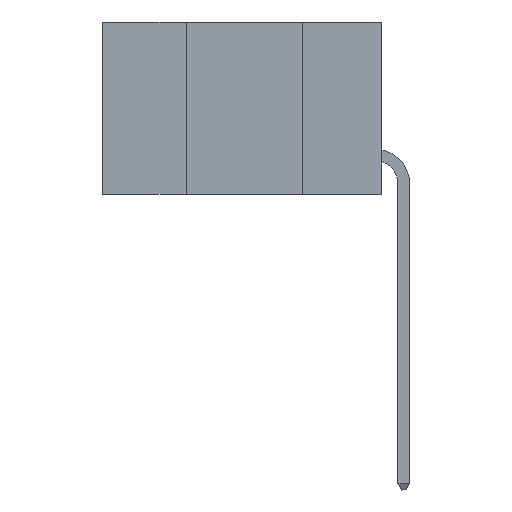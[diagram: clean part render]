
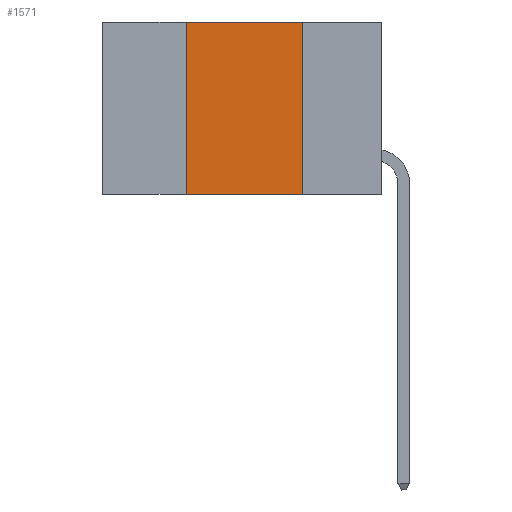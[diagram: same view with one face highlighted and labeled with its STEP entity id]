
A CAD part, left-side view. The second image highlights one B-rep face of the part: STEP entity #1571.
In plain terms, the highlighted planar face has unit normal (-1, 0, 0).
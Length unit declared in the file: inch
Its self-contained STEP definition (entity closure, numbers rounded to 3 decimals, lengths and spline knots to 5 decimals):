
#367 = CARTESIAN_POINT ( 'NONE',  ( 0., 0.6, -0.37 ) ) ;
#556 = VECTOR ( 'NONE', #1005, 39.37008 ) ;
#877 = DIRECTION ( 'NONE',  ( 0., -1., 0. ) ) ;
#901 = PLANE ( 'NONE',  #9043 ) ;
#1005 = DIRECTION ( 'NONE',  ( 0., 0., -1. ) ) ;
#1055 = EDGE_CURVE ( 'NONE', #2250, #11367, #5866, .T. ) ;
#1189 = ORIENTED_EDGE ( 'NONE', *, *, #10576, .F. ) ;
#1543 = ORIENTED_EDGE ( 'NONE', *, *, #1055, .F. ) ;
#1571 = ADVANCED_FACE ( 'NONE', ( #2139 ), #901, .F. ) ;
#1970 = LINE ( 'NONE', #11262, #9979 ) ;
#2139 = FACE_OUTER_BOUND ( 'NONE', #10655, .T. ) ;
#2250 = VERTEX_POINT ( 'NONE', #4619 ) ;
#2549 = ORIENTED_EDGE ( 'NONE', *, *, #5636, .F. ) ;
#2704 = DIRECTION ( 'NONE',  ( 0., 0., -1. ) ) ;
#2835 = VERTEX_POINT ( 'NONE', #10573 ) ;
#3587 = DIRECTION ( 'NONE',  ( 1., 0., 0. ) ) ;
#3677 = CARTESIAN_POINT ( 'NONE',  ( 0., 0.17, 0. ) ) ;
#3863 = LINE ( 'NONE', #10539, #556 ) ;
#4139 = EDGE_CURVE ( 'NONE', #2835, #9492, #4580, .T. ) ;
#4580 = LINE ( 'NONE', #367, #11360 ) ;
#4619 = CARTESIAN_POINT ( 'NONE',  ( 0., 0.42, 0. ) ) ;
#4703 = DIRECTION ( 'NONE',  ( 0., -1., 0. ) ) ;
#5636 = EDGE_CURVE ( 'NONE', #11367, #9492, #3863, .T. ) ;
#5839 = DIRECTION ( 'NONE',  ( 0., 0., 1. ) ) ;
#5866 = LINE ( 'NONE', #7767, #6014 ) ;
#6014 = VECTOR ( 'NONE', #877, 39.37008 ) ;
#6269 = CARTESIAN_POINT ( 'NONE',  ( 0., 0.6, 0. ) ) ;
#6449 = ORIENTED_EDGE ( 'NONE', *, *, #4139, .T. ) ;
#7767 = CARTESIAN_POINT ( 'NONE',  ( 0., 0.6, 0. ) ) ;
#7934 = CARTESIAN_POINT ( 'NONE',  ( 0., 0.17, -0.37 ) ) ;
#9043 = AXIS2_PLACEMENT_3D ( 'NONE', #6269, #3587, #2704 ) ;
#9492 = VERTEX_POINT ( 'NONE', #7934 ) ;
#9979 = VECTOR ( 'NONE', #5839, 39.37008 ) ;
#10539 = CARTESIAN_POINT ( 'NONE',  ( 0., 0.17, 0. ) ) ;
#10573 = CARTESIAN_POINT ( 'NONE',  ( 0., 0.42, -0.37 ) ) ;
#10576 = EDGE_CURVE ( 'NONE', #2835, #2250, #1970, .T. ) ;
#10655 = EDGE_LOOP ( 'NONE', ( #2549, #1543, #1189, #6449 ) ) ;
#11262 = CARTESIAN_POINT ( 'NONE',  ( 0., 0.42, 0. ) ) ;
#11360 = VECTOR ( 'NONE', #4703, 39.37008 ) ;
#11367 = VERTEX_POINT ( 'NONE', #3677 ) ;
